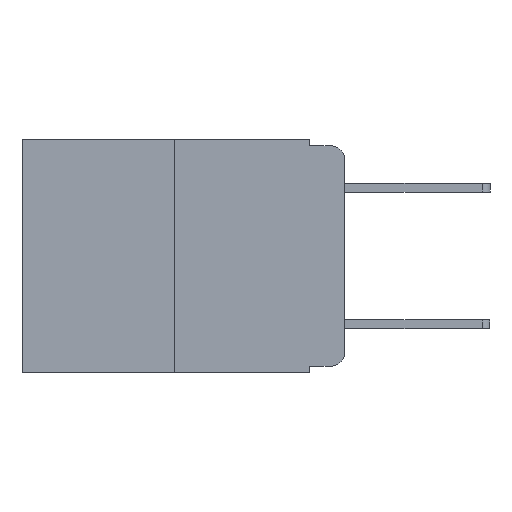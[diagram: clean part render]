
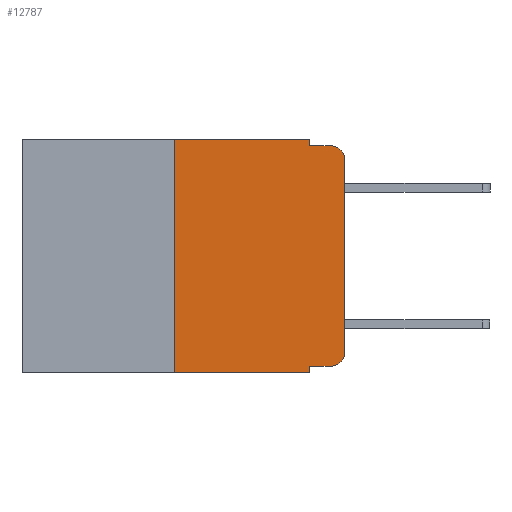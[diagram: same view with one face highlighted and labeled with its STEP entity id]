
A CAD part, left-side view. The second image highlights one B-rep face of the part: STEP entity #12787.
In plain terms, the highlighted planar face has unit normal (-1, 0, 0).
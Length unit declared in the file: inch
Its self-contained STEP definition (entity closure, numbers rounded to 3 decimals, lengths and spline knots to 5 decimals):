
#232 = DIRECTION ( 'NONE',  ( 0., 0., -1. ) ) ;
#391 = CARTESIAN_POINT ( 'NONE',  ( 0., 0., -0.313 ) ) ;
#493 = CARTESIAN_POINT ( 'NONE',  ( 0., 0.051, 0. ) ) ;
#636 = VECTOR ( 'NONE', #9834, 39.37008 ) ;
#930 = VECTOR ( 'NONE', #6542, 39.37008 ) ;
#1917 = CARTESIAN_POINT ( 'NONE',  ( 0., 0.473, -0.343 ) ) ;
#2600 = ORIENTED_EDGE ( 'NONE', *, *, #12180, .F. ) ;
#2702 = LINE ( 'NONE', #8128, #12438 ) ;
#2858 = ORIENTED_EDGE ( 'NONE', *, *, #11523, .F. ) ;
#2936 = LINE ( 'NONE', #5506, #12638 ) ;
#2961 = ORIENTED_EDGE ( 'NONE', *, *, #24881, .F. ) ;
#2984 = CARTESIAN_POINT ( 'NONE',  ( 0., 0.051, -0.333 ) ) ;
#3096 = VECTOR ( 'NONE', #15719, 39.37008 ) ;
#3474 = DIRECTION ( 'NONE',  ( 0., 0., -1. ) ) ;
#3596 = VECTOR ( 'NONE', #11932, 39.37008 ) ;
#4074 = CARTESIAN_POINT ( 'NONE',  ( 0., 0.02, -0.313 ) ) ;
#5343 = EDGE_LOOP ( 'NONE', ( #15278, #13707, #2858, #2961, #7877, #2600, #6617, #14087, #23749, #7318 ) ) ;
#5506 = CARTESIAN_POINT ( 'NONE',  ( 0., 0.051, 0. ) ) ;
#6052 = LINE ( 'NONE', #1917, #636 ) ;
#6075 = DIRECTION ( 'NONE',  ( 0., 0., -1. ) ) ;
#6140 = CARTESIAN_POINT ( 'NONE',  ( 0., 0.051, -0.01 ) ) ;
#6542 = DIRECTION ( 'NONE',  ( 0., 0., 1. ) ) ;
#6617 = ORIENTED_EDGE ( 'NONE', *, *, #17005, .T. ) ;
#6819 = AXIS2_PLACEMENT_3D ( 'NONE', #16027, #21831, #10391 ) ;
#7075 = EDGE_CURVE ( 'NONE', #22828, #21850, #7503, .T. ) ;
#7318 = ORIENTED_EDGE ( 'NONE', *, *, #7075, .T. ) ;
#7503 = CIRCLE ( 'NONE', #15266, 0.02 ) ;
#7877 = ORIENTED_EDGE ( 'NONE', *, *, #10474, .F. ) ;
#8128 = CARTESIAN_POINT ( 'NONE',  ( 0., 0.473, 0. ) ) ;
#8456 = PLANE ( 'NONE',  #6819 ) ;
#9396 = CARTESIAN_POINT ( 'NONE',  ( 0., 0.25, -0.343 ) ) ;
#9440 = VERTEX_POINT ( 'NONE', #16102 ) ;
#9761 = LINE ( 'NONE', #23240, #14218 ) ;
#9834 = DIRECTION ( 'NONE',  ( 0., -1., 0. ) ) ;
#9900 = DIRECTION ( 'NONE',  ( 0., -1., 0. ) ) ;
#10224 = VERTEX_POINT ( 'NONE', #2984 ) ;
#10391 = DIRECTION ( 'NONE',  ( 0., 0., -1. ) ) ;
#10430 = EDGE_CURVE ( 'NONE', #10224, #22828, #9761, .T. ) ;
#10474 = EDGE_CURVE ( 'NONE', #22993, #20993, #2702, .T. ) ;
#10877 = CARTESIAN_POINT ( 'NONE',  ( 0., 0.051, -0.01 ) ) ;
#11228 = CARTESIAN_POINT ( 'NONE',  ( 0., 0.051, 0. ) ) ;
#11523 = EDGE_CURVE ( 'NONE', #21154, #12404, #18968, .T. ) ;
#11693 = FACE_OUTER_BOUND ( 'NONE', #5343, .T. ) ;
#11932 = DIRECTION ( 'NONE',  ( 0., -1., 0. ) ) ;
#12069 = DIRECTION ( 'NONE',  ( -1., 0., 0. ) ) ;
#12180 = EDGE_CURVE ( 'NONE', #20654, #22993, #17076, .T. ) ;
#12404 = VERTEX_POINT ( 'NONE', #14775 ) ;
#12438 = VECTOR ( 'NONE', #23393, 39.37008 ) ;
#12638 = VECTOR ( 'NONE', #3474, 39.37008 ) ;
#12787 = ADVANCED_FACE ( 'NONE', ( #11693 ), #8456, .F. ) ;
#13425 = CIRCLE ( 'NONE', #19171, 0.02 ) ;
#13707 = ORIENTED_EDGE ( 'NONE', *, *, #23028, .T. ) ;
#14007 = EDGE_CURVE ( 'NONE', #21850, #17037, #22969, .T. ) ;
#14087 = ORIENTED_EDGE ( 'NONE', *, *, #17873, .F. ) ;
#14127 = CARTESIAN_POINT ( 'NONE',  ( 0., 0.25, 0. ) ) ;
#14218 = VECTOR ( 'NONE', #9900, 39.37008 ) ;
#14775 = CARTESIAN_POINT ( 'NONE',  ( 0., 0.02, -0.01 ) ) ;
#15266 = AXIS2_PLACEMENT_3D ( 'NONE', #4074, #17520, #6075 ) ;
#15278 = ORIENTED_EDGE ( 'NONE', *, *, #14007, .T. ) ;
#15719 = DIRECTION ( 'NONE',  ( 0., 0., 1. ) ) ;
#16027 = CARTESIAN_POINT ( 'NONE',  ( 0., 0.473, 0. ) ) ;
#16102 = CARTESIAN_POINT ( 'NONE',  ( 0., 0.051, -0.343 ) ) ;
#16213 = VECTOR ( 'NONE', #16969, 39.37008 ) ;
#16969 = DIRECTION ( 'NONE',  ( 0., 0., -1. ) ) ;
#17005 = EDGE_CURVE ( 'NONE', #20654, #9440, #6052, .T. ) ;
#17037 = VERTEX_POINT ( 'NONE', #17482 ) ;
#17076 = LINE ( 'NONE', #14127, #930 ) ;
#17482 = CARTESIAN_POINT ( 'NONE',  ( 0., 0., -0.03 ) ) ;
#17520 = DIRECTION ( 'NONE',  ( -1., 0., 0. ) ) ;
#17873 = EDGE_CURVE ( 'NONE', #10224, #9440, #2936, .T. ) ;
#18968 = LINE ( 'NONE', #6140, #3596 ) ;
#19171 = AXIS2_PLACEMENT_3D ( 'NONE', #23472, #12069, #232 ) ;
#19590 = CARTESIAN_POINT ( 'NONE',  ( 0., 0., 0. ) ) ;
#20654 = VERTEX_POINT ( 'NONE', #9396 ) ;
#20847 = CARTESIAN_POINT ( 'NONE',  ( 0., 0.02, -0.333 ) ) ;
#20993 = VERTEX_POINT ( 'NONE', #493 ) ;
#21154 = VERTEX_POINT ( 'NONE', #10877 ) ;
#21319 = LINE ( 'NONE', #11228, #16213 ) ;
#21426 = CARTESIAN_POINT ( 'NONE',  ( 0., 0.25, 0. ) ) ;
#21831 = DIRECTION ( 'NONE',  ( 1., 0., 0. ) ) ;
#21850 = VERTEX_POINT ( 'NONE', #391 ) ;
#22828 = VERTEX_POINT ( 'NONE', #20847 ) ;
#22969 = LINE ( 'NONE', #19590, #3096 ) ;
#22993 = VERTEX_POINT ( 'NONE', #21426 ) ;
#23028 = EDGE_CURVE ( 'NONE', #17037, #12404, #13425, .T. ) ;
#23240 = CARTESIAN_POINT ( 'NONE',  ( 0., 0.051, -0.333 ) ) ;
#23393 = DIRECTION ( 'NONE',  ( 0., -1., 0. ) ) ;
#23472 = CARTESIAN_POINT ( 'NONE',  ( 0., 0.02, -0.03 ) ) ;
#23749 = ORIENTED_EDGE ( 'NONE', *, *, #10430, .T. ) ;
#24881 = EDGE_CURVE ( 'NONE', #20993, #21154, #21319, .T. ) ;
